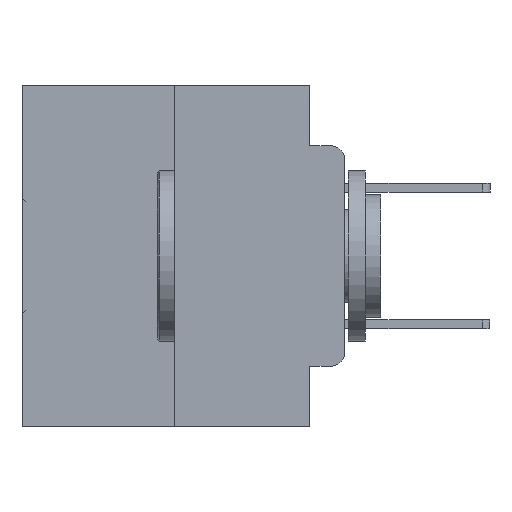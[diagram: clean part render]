
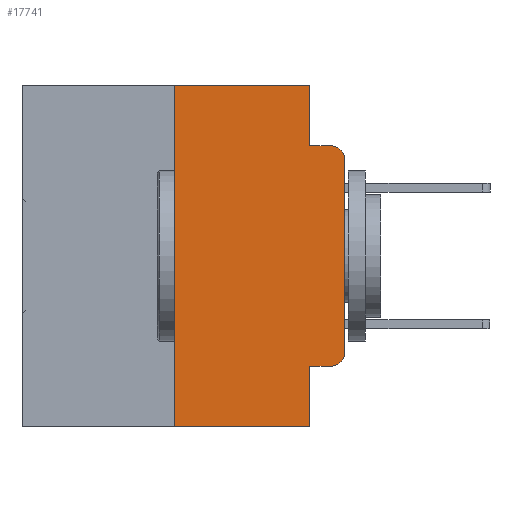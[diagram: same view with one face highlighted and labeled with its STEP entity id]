
A CAD part, left-side view. The second image highlights one B-rep face of the part: STEP entity #17741.
In plain terms, the highlighted planar face has unit normal (-1, 0, 0).
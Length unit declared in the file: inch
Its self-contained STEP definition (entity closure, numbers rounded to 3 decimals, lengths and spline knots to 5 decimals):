
#233 = CARTESIAN_POINT ( 'NONE',  ( 0., 0.473, 0. ) ) ;
#416 = ORIENTED_EDGE ( 'NONE', *, *, #11784, .T. ) ;
#455 = ORIENTED_EDGE ( 'NONE', *, *, #15732, .T. ) ;
#1604 = EDGE_CURVE ( 'NONE', #6763, #8283, #19364, .T. ) ;
#1760 = CARTESIAN_POINT ( 'NONE',  ( 0., 0.02, -0.4115 ) ) ;
#1827 = AXIS2_PLACEMENT_3D ( 'NONE', #19814, #4860, #22246 ) ;
#2468 = DIRECTION ( 'NONE',  ( 0., 0., -1. ) ) ;
#2834 = CARTESIAN_POINT ( 'NONE',  ( 0., 0.473, 0. ) ) ;
#2960 = CARTESIAN_POINT ( 'NONE',  ( 0., 0.25, 0. ) ) ;
#3130 = EDGE_CURVE ( 'NONE', #21648, #24970, #18835, .T. ) ;
#3318 = EDGE_CURVE ( 'NONE', #8283, #28947, #6751, .T. ) ;
#3594 = VECTOR ( 'NONE', #25219, 39.37008 ) ;
#3885 = CARTESIAN_POINT ( 'NONE',  ( 0., 0.02, -0.0885 ) ) ;
#4322 = CARTESIAN_POINT ( 'NONE',  ( 0., 0.051, 0. ) ) ;
#4860 = DIRECTION ( 'NONE',  ( -1., 0., 0. ) ) ;
#5006 = VECTOR ( 'NONE', #23894, 39.37008 ) ;
#5639 = CARTESIAN_POINT ( 'NONE',  ( 0., 0., 0. ) ) ;
#6207 = CIRCLE ( 'NONE', #31078, 0.02 ) ;
#6751 = LINE ( 'NONE', #21702, #12553 ) ;
#6763 = VERTEX_POINT ( 'NONE', #25595 ) ;
#7171 = VECTOR ( 'NONE', #19440, 39.37008 ) ;
#7358 = VERTEX_POINT ( 'NONE', #8280 ) ;
#7482 = CARTESIAN_POINT ( 'NONE',  ( 0., 0.25, -0.5 ) ) ;
#7661 = DIRECTION ( 'NONE',  ( 0., -1., 0. ) ) ;
#8219 = DIRECTION ( 'NONE',  ( 0., 0., 1. ) ) ;
#8280 = CARTESIAN_POINT ( 'NONE',  ( 0., 0.051, -0.4115 ) ) ;
#8283 = VERTEX_POINT ( 'NONE', #19489 ) ;
#8747 = CARTESIAN_POINT ( 'NONE',  ( 0., 0., -0.1085 ) ) ;
#8882 = ORIENTED_EDGE ( 'NONE', *, *, #10141, .T. ) ;
#9067 = CARTESIAN_POINT ( 'NONE',  ( 0., 0.02, -0.1085 ) ) ;
#9466 = VECTOR ( 'NONE', #20360, 39.37008 ) ;
#10141 = EDGE_CURVE ( 'NONE', #24505, #28947, #6207, .T. ) ;
#10408 = ORIENTED_EDGE ( 'NONE', *, *, #1604, .F. ) ;
#10798 = LINE ( 'NONE', #5639, #16629 ) ;
#11533 = DIRECTION ( 'NONE',  ( 0., 0., -1. ) ) ;
#11687 = CARTESIAN_POINT ( 'NONE',  ( 0., 0.051, 0. ) ) ;
#11784 = EDGE_CURVE ( 'NONE', #28730, #24505, #10798, .T. ) ;
#12553 = VECTOR ( 'NONE', #16771, 39.37008 ) ;
#13727 = VECTOR ( 'NONE', #7661, 39.37008 ) ;
#15041 = ORIENTED_EDGE ( 'NONE', *, *, #3130, .T. ) ;
#15473 = DIRECTION ( 'NONE',  ( 0., 0., -1. ) ) ;
#15732 = EDGE_CURVE ( 'NONE', #31499, #28730, #27650, .T. ) ;
#16629 = VECTOR ( 'NONE', #8219, 39.37008 ) ;
#16771 = DIRECTION ( 'NONE',  ( 0., -1., 0. ) ) ;
#17597 = LINE ( 'NONE', #2834, #9466 ) ;
#17741 = ADVANCED_FACE ( 'NONE', ( #27776 ), #27453, .F. ) ;
#18602 = VECTOR ( 'NONE', #2468, 39.37008 ) ;
#18835 = LINE ( 'NONE', #20170, #7171 ) ;
#19364 = LINE ( 'NONE', #4322, #18602 ) ;
#19440 = DIRECTION ( 'NONE',  ( 0., -1., 0. ) ) ;
#19489 = CARTESIAN_POINT ( 'NONE',  ( 0., 0.051, -0.0885 ) ) ;
#19814 = CARTESIAN_POINT ( 'NONE',  ( 0., 0.02, -0.3915 ) ) ;
#19952 = EDGE_CURVE ( 'NONE', #26695, #6763, #17597, .T. ) ;
#20008 = CARTESIAN_POINT ( 'NONE',  ( 0., 0.051, -0.4115 ) ) ;
#20086 = ORIENTED_EDGE ( 'NONE', *, *, #19952, .F. ) ;
#20170 = CARTESIAN_POINT ( 'NONE',  ( 0., 0.473, -0.5 ) ) ;
#20360 = DIRECTION ( 'NONE',  ( 0., -1., 0. ) ) ;
#20406 = CARTESIAN_POINT ( 'NONE',  ( 0., 0., -0.3915 ) ) ;
#21117 = LINE ( 'NONE', #20008, #13727 ) ;
#21648 = VERTEX_POINT ( 'NONE', #7482 ) ;
#21702 = CARTESIAN_POINT ( 'NONE',  ( 0., 0.051, -0.0885 ) ) ;
#22246 = DIRECTION ( 'NONE',  ( 0., 0., -1. ) ) ;
#22311 = EDGE_CURVE ( 'NONE', #7358, #31499, #21117, .T. ) ;
#23396 = LINE ( 'NONE', #2960, #3594 ) ;
#23885 = EDGE_CURVE ( 'NONE', #7358, #24970, #24679, .T. ) ;
#23894 = DIRECTION ( 'NONE',  ( 0., 0., -1. ) ) ;
#24505 = VERTEX_POINT ( 'NONE', #8747 ) ;
#24679 = LINE ( 'NONE', #11687, #5006 ) ;
#24700 = AXIS2_PLACEMENT_3D ( 'NONE', #233, #29838, #15473 ) ;
#24724 = EDGE_LOOP ( 'NONE', ( #416, #8882, #28222, #10408, #20086, #27114, #15041, #28611, #29349, #455 ) ) ;
#24970 = VERTEX_POINT ( 'NONE', #25453 ) ;
#25219 = DIRECTION ( 'NONE',  ( 0., 0., 1. ) ) ;
#25453 = CARTESIAN_POINT ( 'NONE',  ( 0., 0.051, -0.5 ) ) ;
#25595 = CARTESIAN_POINT ( 'NONE',  ( 0., 0.051, 0. ) ) ;
#26109 = DIRECTION ( 'NONE',  ( -1., 0., 0. ) ) ;
#26695 = VERTEX_POINT ( 'NONE', #27284 ) ;
#27114 = ORIENTED_EDGE ( 'NONE', *, *, #31791, .F. ) ;
#27284 = CARTESIAN_POINT ( 'NONE',  ( 0., 0.25, 0. ) ) ;
#27453 = PLANE ( 'NONE',  #24700 ) ;
#27650 = CIRCLE ( 'NONE', #1827, 0.02 ) ;
#27776 = FACE_OUTER_BOUND ( 'NONE', #24724, .T. ) ;
#28222 = ORIENTED_EDGE ( 'NONE', *, *, #3318, .F. ) ;
#28611 = ORIENTED_EDGE ( 'NONE', *, *, #23885, .F. ) ;
#28730 = VERTEX_POINT ( 'NONE', #20406 ) ;
#28947 = VERTEX_POINT ( 'NONE', #3885 ) ;
#29349 = ORIENTED_EDGE ( 'NONE', *, *, #22311, .T. ) ;
#29838 = DIRECTION ( 'NONE',  ( 1., 0., 0. ) ) ;
#31078 = AXIS2_PLACEMENT_3D ( 'NONE', #9067, #26109, #11533 ) ;
#31499 = VERTEX_POINT ( 'NONE', #1760 ) ;
#31791 = EDGE_CURVE ( 'NONE', #21648, #26695, #23396, .T. ) ;
